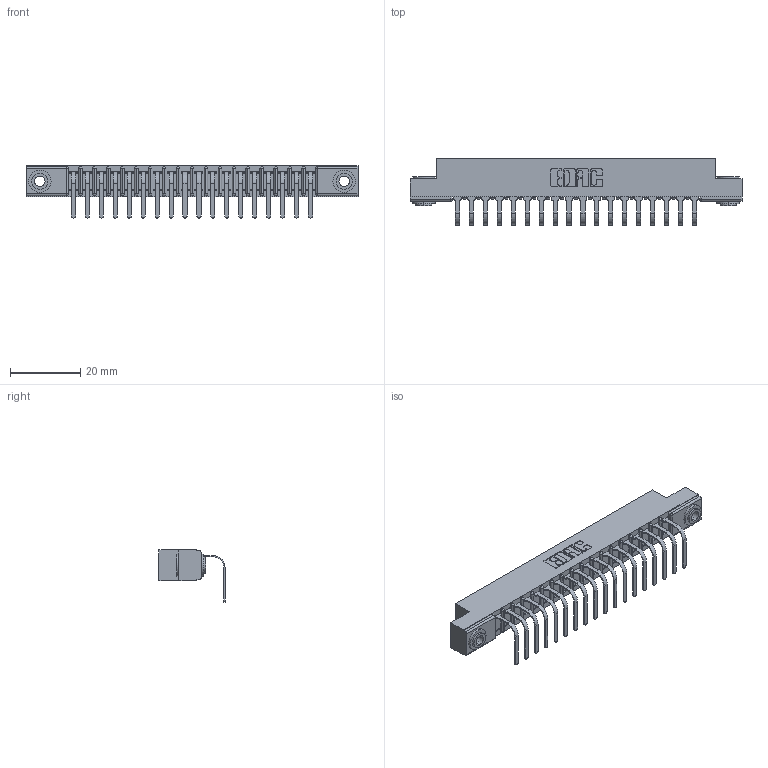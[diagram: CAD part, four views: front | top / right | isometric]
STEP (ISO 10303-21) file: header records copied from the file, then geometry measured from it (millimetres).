
FILE_DESCRIPTION (( 'STEP AP203' ), '1' );
FILE_NAME ('357-018-458-103.STEP', '2022-07-18T22:53:07', ( '' ), ( '' ), 'SwSTEP 2.0', 'SolidWorks 2020', '' );
FILE_SCHEMA (( 'CONFIG_CONTROL_DESIGN' ));
Length unit declared in the file: inch
Products named in the file (4): 307-290-001_558 - 2 (Single); 307 Part_.156 Dia Mounting Holes; 345-250-002_345-250-002-102; 357-018-458-103
Assembly tree (21 placements, depth 2):
  357-018-458-103
    307 Part_.156 Dia Mounting Holes
    307-290-001_558 - 2 (Single)  x18
    345-250-002_345-250-002-102  x2
Bounding box: 94.34 x 18.78 x 14.81 mm (x, y, z)
Volume: 6041.4 mm3; surface area: 9916.2 mm2
Topology: 21 solids, 21 shells, 1269 faces, 3567 edges, 2298 vertices
Faces by surface type: plane 796, cylinder 427, sphere 38, cone 8
Entity records: 19559 total; most frequent: CARTESIAN_POINT 3265, ORIENTED_EDGE 3242, DIRECTION 3205, EDGE_CURVE 1621, VECTOR 1225, LINE 1225, VERTEX_POINT 1050, AXIS2_PLACEMENT_3D 990
